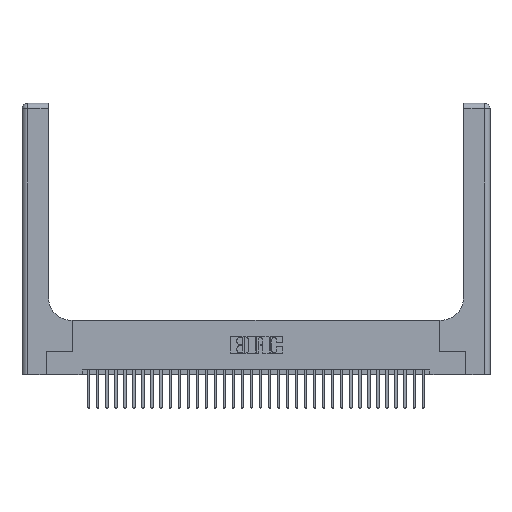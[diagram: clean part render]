
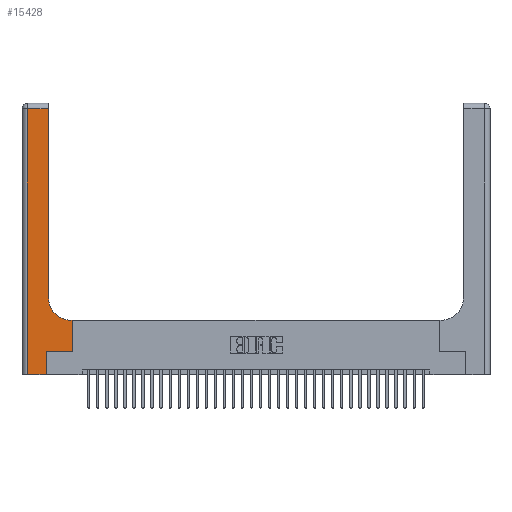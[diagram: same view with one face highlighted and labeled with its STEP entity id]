
A CAD part, top view. The second image highlights one B-rep face of the part: STEP entity #15428.
In plain terms, the highlighted planar face has unit normal (0, 0, 1).
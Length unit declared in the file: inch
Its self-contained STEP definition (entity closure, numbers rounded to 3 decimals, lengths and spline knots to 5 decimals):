
#634 = EDGE_LOOP ( 'NONE', ( #20409, #25120, #14826, #33948, #5679, #23186, #17473, #32114, #8531 ) ) ;
#770 = CARTESIAN_POINT ( 'NONE',  ( 0.2915, 3., 0.37 ) ) ;
#1531 = CARTESIAN_POINT ( 'NONE',  ( 0.5585, 0.25, 0.37 ) ) ;
#1881 = EDGE_CURVE ( 'NONE', #29329, #32477, #20051, .T. ) ;
#1905 = DIRECTION ( 'NONE',  ( 1., 0., 0. ) ) ;
#2132 = CARTESIAN_POINT ( 'NONE',  ( 0.5415, 0.85, 0.37 ) ) ;
#3451 = EDGE_CURVE ( 'NONE', #20252, #6869, #22937, .T. ) ;
#3735 = CARTESIAN_POINT ( 'NONE',  ( 0.06, 2.94, 0.37 ) ) ;
#3765 = LINE ( 'NONE', #34532, #29080 ) ;
#3928 = CARTESIAN_POINT ( 'NONE',  ( 0., 3., 0.37 ) ) ;
#4508 = DIRECTION ( 'NONE',  ( -1., 0., 0. ) ) ;
#4581 = VECTOR ( 'NONE', #11220, 39.37008 ) ;
#5679 = ORIENTED_EDGE ( 'NONE', *, *, #10115, .T. ) ;
#6766 = CARTESIAN_POINT ( 'NONE',  ( 0.269, 0.25, 0.37 ) ) ;
#6869 = VERTEX_POINT ( 'NONE', #28124 ) ;
#7847 = EDGE_CURVE ( 'NONE', #9870, #14353, #15937, .T. ) ;
#8505 = VERTEX_POINT ( 'NONE', #29535 ) ;
#8531 = ORIENTED_EDGE ( 'NONE', *, *, #14977, .T. ) ;
#8858 = VECTOR ( 'NONE', #34983, 39.37008 ) ;
#9219 = EDGE_CURVE ( 'NONE', #6869, #26701, #32554, .T. ) ;
#9395 = VERTEX_POINT ( 'NONE', #12563 ) ;
#9773 = DIRECTION ( 'NONE',  ( 1., 0., 0. ) ) ;
#9870 = VERTEX_POINT ( 'NONE', #1531 ) ;
#9902 = DIRECTION ( 'NONE',  ( -1., 0., 0. ) ) ;
#10115 = EDGE_CURVE ( 'NONE', #32477, #8505, #11017, .T. ) ;
#11017 = LINE ( 'NONE', #35100, #8858 ) ;
#11220 = DIRECTION ( 'NONE',  ( 1., 0., 0. ) ) ;
#12563 = CARTESIAN_POINT ( 'NONE',  ( 0.5415, 0.6, 0.37 ) ) ;
#12671 = EDGE_CURVE ( 'NONE', #26701, #29329, #28743, .T. ) ;
#13087 = CARTESIAN_POINT ( 'NONE',  ( 0.2915, 0.85, 0.37 ) ) ;
#13471 = DIRECTION ( 'NONE',  ( 0., 0., -1. ) ) ;
#13665 = VECTOR ( 'NONE', #34258, 39.37008 ) ;
#13905 = VECTOR ( 'NONE', #31020, 39.37008 ) ;
#14171 = VECTOR ( 'NONE', #17254, 39.37008 ) ;
#14353 = VERTEX_POINT ( 'NONE', #15742 ) ;
#14826 = ORIENTED_EDGE ( 'NONE', *, *, #12671, .T. ) ;
#14977 = EDGE_CURVE ( 'NONE', #9395, #20252, #34263, .T. ) ;
#15428 = ADVANCED_FACE ( 'NONE', ( #34164 ), #28497, .F. ) ;
#15742 = CARTESIAN_POINT ( 'NONE',  ( 0.5585, 0.6, 0.37 ) ) ;
#15937 = LINE ( 'NONE', #21668, #26181 ) ;
#15992 = LINE ( 'NONE', #6766, #34854 ) ;
#16569 = AXIS2_PLACEMENT_3D ( 'NONE', #2132, #13471, #1905 ) ;
#17254 = DIRECTION ( 'NONE',  ( 0., -1., 0. ) ) ;
#17422 = EDGE_CURVE ( 'NONE', #8505, #9870, #15992, .T. ) ;
#17473 = ORIENTED_EDGE ( 'NONE', *, *, #7847, .T. ) ;
#20051 = LINE ( 'NONE', #23379, #4581 ) ;
#20252 = VERTEX_POINT ( 'NONE', #13087 ) ;
#20409 = ORIENTED_EDGE ( 'NONE', *, *, #3451, .T. ) ;
#21668 = CARTESIAN_POINT ( 'NONE',  ( 0.5585, 0.25, 0.37 ) ) ;
#21754 = CARTESIAN_POINT ( 'NONE',  ( 0.06, 0., 0.37 ) ) ;
#22937 = LINE ( 'NONE', #770, #13905 ) ;
#23026 = CARTESIAN_POINT ( 'NONE',  ( 0.269, 0., 0.37 ) ) ;
#23186 = ORIENTED_EDGE ( 'NONE', *, *, #17422, .T. ) ;
#23379 = CARTESIAN_POINT ( 'NONE',  ( 0., 0., 0.37 ) ) ;
#25120 = ORIENTED_EDGE ( 'NONE', *, *, #9219, .T. ) ;
#26181 = VECTOR ( 'NONE', #26746, 39.37008 ) ;
#26701 = VERTEX_POINT ( 'NONE', #3735 ) ;
#26746 = DIRECTION ( 'NONE',  ( 0., 1., 0. ) ) ;
#26762 = DIRECTION ( 'NONE',  ( 0., 0., -1. ) ) ;
#28124 = CARTESIAN_POINT ( 'NONE',  ( 0.2915, 2.94, 0.37 ) ) ;
#28423 = EDGE_CURVE ( 'NONE', #14353, #9395, #3765, .T. ) ;
#28471 = CARTESIAN_POINT ( 'NONE',  ( 0., 2.94, 0.37 ) ) ;
#28497 = PLANE ( 'NONE',  #33519 ) ;
#28743 = LINE ( 'NONE', #29938, #14171 ) ;
#29080 = VECTOR ( 'NONE', #9902, 39.37008 ) ;
#29329 = VERTEX_POINT ( 'NONE', #21754 ) ;
#29535 = CARTESIAN_POINT ( 'NONE',  ( 0.269, 0.25, 0.37 ) ) ;
#29938 = CARTESIAN_POINT ( 'NONE',  ( 0.06, 3., 0.37 ) ) ;
#31020 = DIRECTION ( 'NONE',  ( 0., 1., 0. ) ) ;
#32114 = ORIENTED_EDGE ( 'NONE', *, *, #28423, .T. ) ;
#32477 = VERTEX_POINT ( 'NONE', #23026 ) ;
#32554 = LINE ( 'NONE', #28471, #13665 ) ;
#33519 = AXIS2_PLACEMENT_3D ( 'NONE', #3928, #26762, #4508 ) ;
#33948 = ORIENTED_EDGE ( 'NONE', *, *, #1881, .T. ) ;
#34164 = FACE_OUTER_BOUND ( 'NONE', #634, .T. ) ;
#34258 = DIRECTION ( 'NONE',  ( -1., 0., 0. ) ) ;
#34263 = CIRCLE ( 'NONE', #16569, 0.25 ) ;
#34532 = CARTESIAN_POINT ( 'NONE',  ( 0.2915, 0.6, 0.37 ) ) ;
#34854 = VECTOR ( 'NONE', #9773, 39.37008 ) ;
#34983 = DIRECTION ( 'NONE',  ( 0., 1., 0. ) ) ;
#35100 = CARTESIAN_POINT ( 'NONE',  ( 0.269, 0., 0.37 ) ) ;
